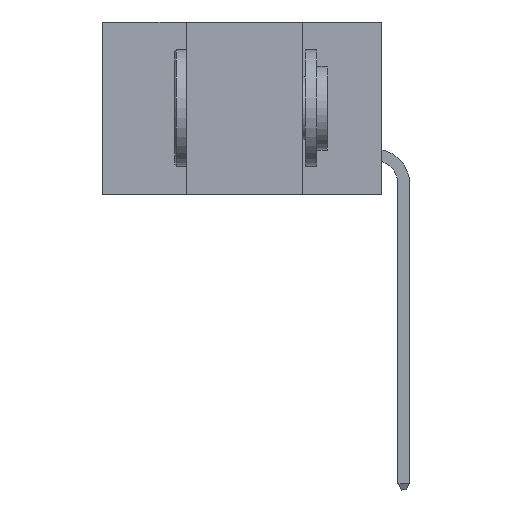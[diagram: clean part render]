
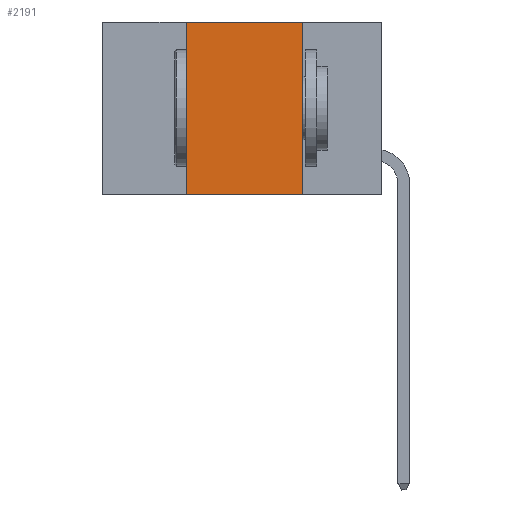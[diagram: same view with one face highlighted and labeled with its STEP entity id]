
A CAD part, left-side view. The second image highlights one B-rep face of the part: STEP entity #2191.
In plain terms, the highlighted planar face has unit normal (-1, 0, 0).
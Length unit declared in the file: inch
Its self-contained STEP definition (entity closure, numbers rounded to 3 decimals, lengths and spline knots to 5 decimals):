
#1634 = VECTOR ( 'NONE', #3566, 39.37008 ) ;
#1738 = FACE_OUTER_BOUND ( 'NONE', #2044, .T. ) ;
#2044 = EDGE_LOOP ( 'NONE', ( #2622, #12108, #20183, #16750 ) ) ;
#2159 = CARTESIAN_POINT ( 'NONE',  ( 0., 0.6, -0.37 ) ) ;
#2191 = ADVANCED_FACE ( 'NONE', ( #1738 ), #5011, .F. ) ;
#2371 = VECTOR ( 'NONE', #4418, 39.37008 ) ;
#2622 = ORIENTED_EDGE ( 'NONE', *, *, #19626, .F. ) ;
#3368 = LINE ( 'NONE', #14096, #2371 ) ;
#3566 = DIRECTION ( 'NONE',  ( 0., -1., 0. ) ) ;
#4418 = DIRECTION ( 'NONE',  ( 0., 0., 1. ) ) ;
#4563 = CARTESIAN_POINT ( 'NONE',  ( 0., 0.42, -0.37 ) ) ;
#5011 = PLANE ( 'NONE',  #5937 ) ;
#5079 = EDGE_CURVE ( 'NONE', #16432, #11591, #9723, .T. ) ;
#5613 = CARTESIAN_POINT ( 'NONE',  ( 0., 0.17, 0. ) ) ;
#5937 = AXIS2_PLACEMENT_3D ( 'NONE', #19387, #17861, #19460 ) ;
#7254 = CARTESIAN_POINT ( 'NONE',  ( 0., 0.42, 0. ) ) ;
#7325 = CARTESIAN_POINT ( 'NONE',  ( 0., 0.6, 0. ) ) ;
#9723 = LINE ( 'NONE', #2159, #1634 ) ;
#11591 = VERTEX_POINT ( 'NONE', #17220 ) ;
#12018 = VECTOR ( 'NONE', #18517, 39.37008 ) ;
#12108 = ORIENTED_EDGE ( 'NONE', *, *, #19190, .F. ) ;
#13644 = CARTESIAN_POINT ( 'NONE',  ( 0., 0.17, 0. ) ) ;
#14096 = CARTESIAN_POINT ( 'NONE',  ( 0., 0.42, 0. ) ) ;
#16432 = VERTEX_POINT ( 'NONE', #4563 ) ;
#16750 = ORIENTED_EDGE ( 'NONE', *, *, #5079, .T. ) ;
#16797 = VECTOR ( 'NONE', #20031, 39.37008 ) ;
#17220 = CARTESIAN_POINT ( 'NONE',  ( 0., 0.17, -0.37 ) ) ;
#17480 = VERTEX_POINT ( 'NONE', #5613 ) ;
#17783 = LINE ( 'NONE', #13644, #16797 ) ;
#17861 = DIRECTION ( 'NONE',  ( 1., 0., 0. ) ) ;
#18383 = EDGE_CURVE ( 'NONE', #16432, #20336, #3368, .T. ) ;
#18517 = DIRECTION ( 'NONE',  ( 0., -1., 0. ) ) ;
#19190 = EDGE_CURVE ( 'NONE', #20336, #17480, #20468, .T. ) ;
#19387 = CARTESIAN_POINT ( 'NONE',  ( 0., 0.6, 0. ) ) ;
#19460 = DIRECTION ( 'NONE',  ( 0., 0., -1. ) ) ;
#19626 = EDGE_CURVE ( 'NONE', #17480, #11591, #17783, .T. ) ;
#20031 = DIRECTION ( 'NONE',  ( 0., 0., -1. ) ) ;
#20183 = ORIENTED_EDGE ( 'NONE', *, *, #18383, .F. ) ;
#20336 = VERTEX_POINT ( 'NONE', #7254 ) ;
#20468 = LINE ( 'NONE', #7325, #12018 ) ;
